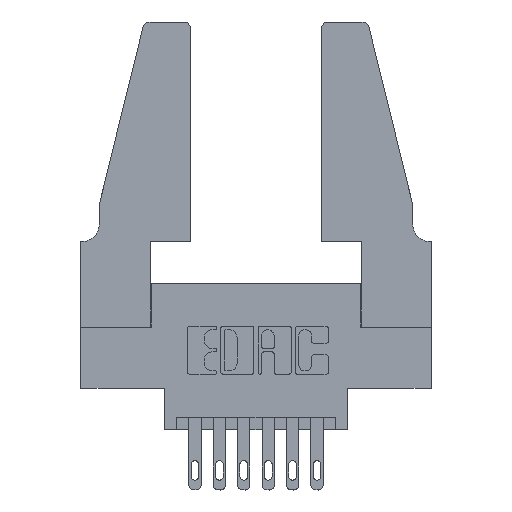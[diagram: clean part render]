
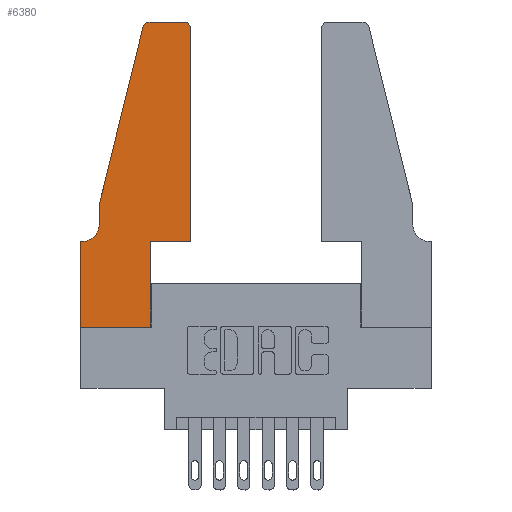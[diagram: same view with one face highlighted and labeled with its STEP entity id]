
A CAD part, top view. The second image highlights one B-rep face of the part: STEP entity #6380.
In plain terms, the highlighted planar face has unit normal (0, 0, 1).
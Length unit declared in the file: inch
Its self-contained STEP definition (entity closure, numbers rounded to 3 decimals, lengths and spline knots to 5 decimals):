
#52 = DIRECTION ( 'NONE',  ( 1., 0., 0. ) ) ;
#264 = EDGE_CURVE ( 'NONE', #6202, #438, #10920, .T. ) ;
#438 = VERTEX_POINT ( 'NONE', #6294 ) ;
#585 = LINE ( 'NONE', #1207, #11705 ) ;
#668 = EDGE_CURVE ( 'NONE', #3963, #2889, #4384, .T. ) ;
#711 = CARTESIAN_POINT ( 'NONE',  ( 0.2865, 0.35, 0.37 ) ) ;
#760 = AXIS2_PLACEMENT_3D ( 'NONE', #7220, #6188, #8900 ) ;
#883 = VERTEX_POINT ( 'NONE', #4897 ) ;
#1035 = CIRCLE ( 'NONE', #11387, 0.07 ) ;
#1086 = FACE_OUTER_BOUND ( 'NONE', #10638, .T. ) ;
#1149 = VERTEX_POINT ( 'NONE', #2631 ) ;
#1183 = LINE ( 'NONE', #6595, #6031 ) ;
#1207 = CARTESIAN_POINT ( 'NONE',  ( 0.0755, 0.5, 0.37 ) ) ;
#1346 = CARTESIAN_POINT ( 'NONE',  ( 0., 0.35, 0.37 ) ) ;
#1387 = DIRECTION ( 'NONE',  ( 0., 0., 1. ) ) ;
#1583 = CARTESIAN_POINT ( 'NONE',  ( 0., 0., 0.37 ) ) ;
#1843 = CARTESIAN_POINT ( 'NONE',  ( 0.4205, 1.25, 0.37 ) ) ;
#2191 = VERTEX_POINT ( 'NONE', #9793 ) ;
#2302 = VECTOR ( 'NONE', #2972, 39.37008 ) ;
#2321 = VECTOR ( 'NONE', #52, 39.37008 ) ;
#2446 = ORIENTED_EDGE ( 'NONE', *, *, #668, .T. ) ;
#2631 = CARTESIAN_POINT ( 'NONE',  ( 0., 0.35, 0.37 ) ) ;
#2889 = VERTEX_POINT ( 'NONE', #5773 ) ;
#2972 = DIRECTION ( 'NONE',  ( 1., 0., 0. ) ) ;
#3027 = AXIS2_PLACEMENT_3D ( 'NONE', #1346, #1387, #7756 ) ;
#3043 = EDGE_CURVE ( 'NONE', #10090, #9557, #8292, .T. ) ;
#3147 = EDGE_CURVE ( 'NONE', #3769, #2191, #1035, .T. ) ;
#3195 = DIRECTION ( 'NONE',  ( 1., 0., 0. ) ) ;
#3203 = EDGE_CURVE ( 'NONE', #8123, #883, #585, .T. ) ;
#3358 = EDGE_CURVE ( 'NONE', #5541, #6202, #11443, .T. ) ;
#3746 = CIRCLE ( 'NONE', #760, 0.03 ) ;
#3769 = VERTEX_POINT ( 'NONE', #10762 ) ;
#3963 = VERTEX_POINT ( 'NONE', #6160 ) ;
#3975 = CARTESIAN_POINT ( 'NONE',  ( 0.4505, 0.35, 0.37 ) ) ;
#4013 = ORIENTED_EDGE ( 'NONE', *, *, #9256, .T. ) ;
#4032 = CARTESIAN_POINT ( 'NONE',  ( 0.284, 1.22, 0.37 ) ) ;
#4266 = ORIENTED_EDGE ( 'NONE', *, *, #3043, .T. ) ;
#4346 = VECTOR ( 'NONE', #9527, 39.37008 ) ;
#4384 = LINE ( 'NONE', #10473, #6073 ) ;
#4604 = AXIS2_PLACEMENT_3D ( 'NONE', #4032, #5009, #3195 ) ;
#4897 = CARTESIAN_POINT ( 'NONE',  ( 0.0755, 0.5, 0.37 ) ) ;
#5009 = DIRECTION ( 'NONE',  ( 0., 0., 1. ) ) ;
#5046 = LINE ( 'NONE', #1583, #5321 ) ;
#5321 = VECTOR ( 'NONE', #7996, 39.37008 ) ;
#5348 = DIRECTION ( 'NONE',  ( -1., 0., 0. ) ) ;
#5437 = VECTOR ( 'NONE', #7877, 39.37008 ) ;
#5541 = VERTEX_POINT ( 'NONE', #8700 ) ;
#5652 = ORIENTED_EDGE ( 'NONE', *, *, #3147, .T. ) ;
#5773 = CARTESIAN_POINT ( 'NONE',  ( 0.4505, 1.22, 0.37 ) ) ;
#6031 = VECTOR ( 'NONE', #7508, 39.37008 ) ;
#6073 = VECTOR ( 'NONE', #9610, 39.37008 ) ;
#6153 = LINE ( 'NONE', #3975, #2302 ) ;
#6160 = CARTESIAN_POINT ( 'NONE',  ( 0.4505, 0.35, 0.37 ) ) ;
#6188 = DIRECTION ( 'NONE',  ( 0., 0., 1. ) ) ;
#6202 = VERTEX_POINT ( 'NONE', #6644 ) ;
#6294 = CARTESIAN_POINT ( 'NONE',  ( 0.2865, 0.35, 0.37 ) ) ;
#6380 = ADVANCED_FACE ( 'NONE', ( #1086 ), #11334, .T. ) ;
#6595 = CARTESIAN_POINT ( 'NONE',  ( 0.0755, 0.5, 0.37 ) ) ;
#6644 = CARTESIAN_POINT ( 'NONE',  ( 0.2865, 0., 0.37 ) ) ;
#6932 = CARTESIAN_POINT ( 'NONE',  ( 0.0755, 0.35, 0.37 ) ) ;
#7220 = CARTESIAN_POINT ( 'NONE',  ( 0.4205, 1.22, 0.37 ) ) ;
#7508 = DIRECTION ( 'NONE',  ( 0., -1., 0. ) ) ;
#7756 = DIRECTION ( 'NONE',  ( 1., 0., 0. ) ) ;
#7835 = EDGE_CURVE ( 'NONE', #2191, #1149, #9613, .T. ) ;
#7877 = DIRECTION ( 'NONE',  ( -1., 0., 0. ) ) ;
#7920 = CARTESIAN_POINT ( 'NONE',  ( 0.2605, 1.25, 0.37 ) ) ;
#7980 = ORIENTED_EDGE ( 'NONE', *, *, #10368, .T. ) ;
#7996 = DIRECTION ( 'NONE',  ( 0., -1., 0. ) ) ;
#8052 = CIRCLE ( 'NONE', #4604, 0.03 ) ;
#8088 = VECTOR ( 'NONE', #11741, 39.37008 ) ;
#8112 = DIRECTION ( 'NONE',  ( 0., 0., -1. ) ) ;
#8123 = VERTEX_POINT ( 'NONE', #8202 ) ;
#8202 = CARTESIAN_POINT ( 'NONE',  ( 0.25487, 1.22718, 0.37 ) ) ;
#8292 = LINE ( 'NONE', #7920, #5437 ) ;
#8397 = EDGE_CURVE ( 'NONE', #883, #3769, #1183, .T. ) ;
#8700 = CARTESIAN_POINT ( 'NONE',  ( 0., 0., 0.37 ) ) ;
#8900 = DIRECTION ( 'NONE',  ( 1., 0., 0. ) ) ;
#8956 = ORIENTED_EDGE ( 'NONE', *, *, #10572, .T. ) ;
#9063 = EDGE_CURVE ( 'NONE', #438, #3963, #6153, .T. ) ;
#9067 = CARTESIAN_POINT ( 'NONE',  ( 0.0055, 0.42, 0.37 ) ) ;
#9095 = CARTESIAN_POINT ( 'NONE',  ( 0., 0., 0.37 ) ) ;
#9256 = EDGE_CURVE ( 'NONE', #2889, #10090, #3746, .T. ) ;
#9395 = CARTESIAN_POINT ( 'NONE',  ( 0.284, 1.25, 0.37 ) ) ;
#9527 = DIRECTION ( 'NONE',  ( -1., 0., 0. ) ) ;
#9557 = VERTEX_POINT ( 'NONE', #9395 ) ;
#9610 = DIRECTION ( 'NONE',  ( 0., 1., 0. ) ) ;
#9613 = LINE ( 'NONE', #6932, #4346 ) ;
#9734 = DIRECTION ( 'NONE',  ( -0.239, -0.971, 0. ) ) ;
#9793 = CARTESIAN_POINT ( 'NONE',  ( 0.0055, 0.35, 0.37 ) ) ;
#10090 = VERTEX_POINT ( 'NONE', #1843 ) ;
#10125 = ORIENTED_EDGE ( 'NONE', *, *, #3203, .T. ) ;
#10368 = EDGE_CURVE ( 'NONE', #9557, #8123, #8052, .T. ) ;
#10473 = CARTESIAN_POINT ( 'NONE',  ( 0.4505, 0.35, 0.37 ) ) ;
#10530 = ORIENTED_EDGE ( 'NONE', *, *, #9063, .T. ) ;
#10572 = EDGE_CURVE ( 'NONE', #1149, #5541, #5046, .T. ) ;
#10580 = ORIENTED_EDGE ( 'NONE', *, *, #3358, .T. ) ;
#10638 = EDGE_LOOP ( 'NONE', ( #4266, #7980, #10125, #11480, #5652, #10869, #8956, #10580, #11130, #10530, #2446, #4013 ) ) ;
#10762 = CARTESIAN_POINT ( 'NONE',  ( 0.0755, 0.42, 0.37 ) ) ;
#10869 = ORIENTED_EDGE ( 'NONE', *, *, #7835, .T. ) ;
#10920 = LINE ( 'NONE', #711, #8088 ) ;
#11130 = ORIENTED_EDGE ( 'NONE', *, *, #264, .T. ) ;
#11334 = PLANE ( 'NONE',  #3027 ) ;
#11387 = AXIS2_PLACEMENT_3D ( 'NONE', #9067, #8112, #5348 ) ;
#11443 = LINE ( 'NONE', #9095, #2321 ) ;
#11480 = ORIENTED_EDGE ( 'NONE', *, *, #8397, .T. ) ;
#11705 = VECTOR ( 'NONE', #9734, 39.37008 ) ;
#11741 = DIRECTION ( 'NONE',  ( 0., 1., 0. ) ) ;
